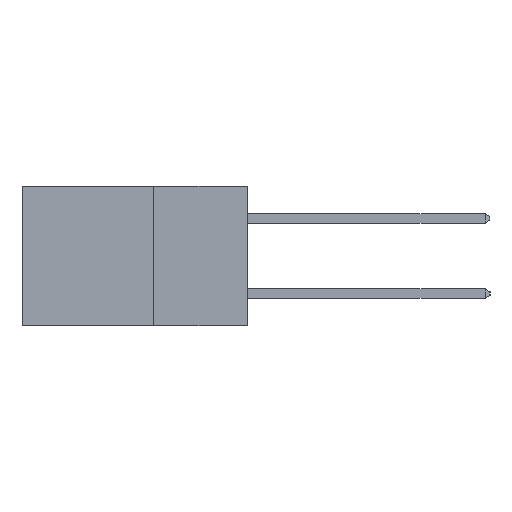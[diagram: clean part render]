
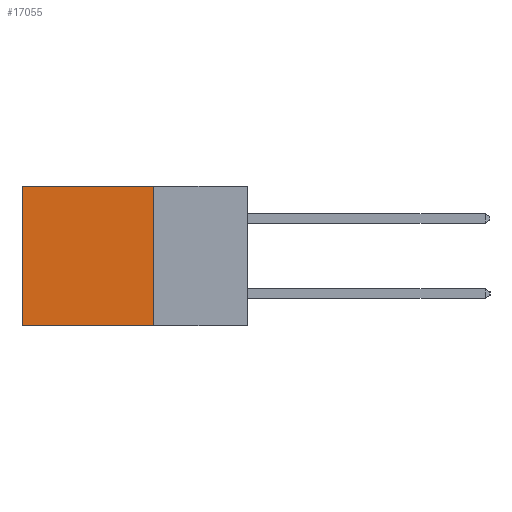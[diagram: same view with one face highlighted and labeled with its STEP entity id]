
A CAD part, left-side view. The second image highlights one B-rep face of the part: STEP entity #17055.
In plain terms, the highlighted planar face has unit normal (-1, 0, 0).
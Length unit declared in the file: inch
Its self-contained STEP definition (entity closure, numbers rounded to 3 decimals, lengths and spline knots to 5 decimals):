
#992 = CARTESIAN_POINT ( 'NONE',  ( 0.2615, 0.25, -0.37 ) ) ;
#1396 = ORIENTED_EDGE ( 'NONE', *, *, #6467, .T. ) ;
#1708 = ORIENTED_EDGE ( 'NONE', *, *, #6722, .T. ) ;
#2145 = CARTESIAN_POINT ( 'NONE',  ( 0.2615, 0.6, 0. ) ) ;
#3876 = CARTESIAN_POINT ( 'NONE',  ( 0.2615, 0.25, 0. ) ) ;
#3920 = VERTEX_POINT ( 'NONE', #3876 ) ;
#4318 = EDGE_CURVE ( 'NONE', #3920, #24468, #9941, .T. ) ;
#4938 = VECTOR ( 'NONE', #21471, 39.37008 ) ;
#5235 = CARTESIAN_POINT ( 'NONE',  ( 0.2615, 0.6, -0.37 ) ) ;
#5266 = EDGE_LOOP ( 'NONE', ( #1708, #15697, #23208, #1396 ) ) ;
#6467 = EDGE_CURVE ( 'NONE', #3920, #16473, #21852, .T. ) ;
#6530 = DIRECTION ( 'NONE',  ( 0., 0., -1. ) ) ;
#6722 = EDGE_CURVE ( 'NONE', #16473, #12041, #15265, .T. ) ;
#8193 = DIRECTION ( 'NONE',  ( 0., 1., 0. ) ) ;
#8768 = FACE_OUTER_BOUND ( 'NONE', #5266, .T. ) ;
#9941 = LINE ( 'NONE', #992, #20775 ) ;
#11226 = VECTOR ( 'NONE', #8193, 39.37008 ) ;
#11235 = CARTESIAN_POINT ( 'NONE',  ( 0.2615, 0.25, 0. ) ) ;
#12041 = VERTEX_POINT ( 'NONE', #5235 ) ;
#12288 = PLANE ( 'NONE',  #20374 ) ;
#13861 = CARTESIAN_POINT ( 'NONE',  ( 0.2615, 0.6, -0.37 ) ) ;
#15265 = LINE ( 'NONE', #13861, #4938 ) ;
#15697 = ORIENTED_EDGE ( 'NONE', *, *, #16519, .F. ) ;
#16385 = LINE ( 'NONE', #21651, #11226 ) ;
#16473 = VERTEX_POINT ( 'NONE', #2145 ) ;
#16519 = EDGE_CURVE ( 'NONE', #24468, #12041, #16385, .T. ) ;
#16652 = DIRECTION ( 'NONE',  ( 0., 0., -1. ) ) ;
#17055 = ADVANCED_FACE ( 'NONE', ( #8768 ), #12288, .F. ) ;
#17390 = VECTOR ( 'NONE', #22727, 39.37008 ) ;
#18119 = DIRECTION ( 'NONE',  ( 1., 0., 0. ) ) ;
#20374 = AXIS2_PLACEMENT_3D ( 'NONE', #23779, #18119, #6530 ) ;
#20439 = CARTESIAN_POINT ( 'NONE',  ( 0.2615, 0.25, -0.37 ) ) ;
#20775 = VECTOR ( 'NONE', #16652, 39.37008 ) ;
#21471 = DIRECTION ( 'NONE',  ( 0., 0., -1. ) ) ;
#21651 = CARTESIAN_POINT ( 'NONE',  ( 0.2615, 0.25, -0.37 ) ) ;
#21852 = LINE ( 'NONE', #11235, #17390 ) ;
#22727 = DIRECTION ( 'NONE',  ( 0., 1., 0. ) ) ;
#23208 = ORIENTED_EDGE ( 'NONE', *, *, #4318, .F. ) ;
#23779 = CARTESIAN_POINT ( 'NONE',  ( 0.2615, 0.25, -0.37 ) ) ;
#24468 = VERTEX_POINT ( 'NONE', #20439 ) ;
